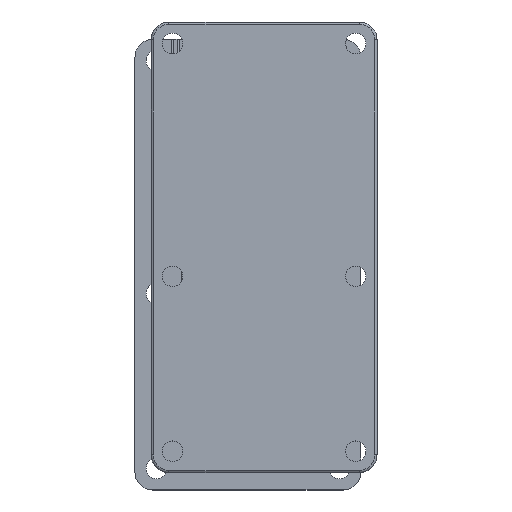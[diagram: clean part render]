
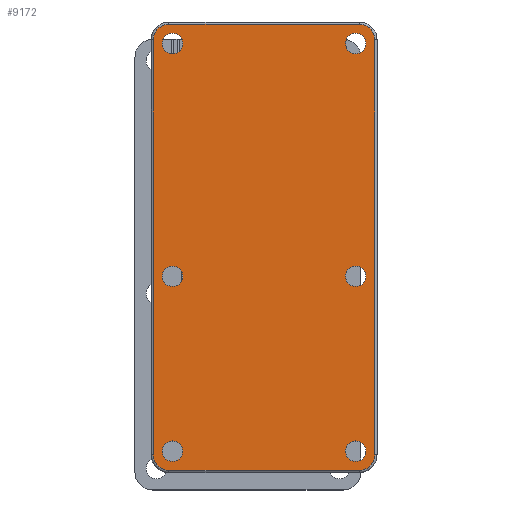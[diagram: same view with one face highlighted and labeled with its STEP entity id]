
A CAD part, top view. The second image highlights one B-rep face of the part: STEP entity #9172.
In plain terms, the highlighted planar face has unit normal (0, 0, 1).
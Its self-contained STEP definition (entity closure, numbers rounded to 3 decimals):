
#223=FACE_BOUND('',#3363,.T.);
#224=FACE_BOUND('',#3364,.T.);
#225=FACE_BOUND('',#3365,.T.);
#226=FACE_BOUND('',#3366,.T.);
#227=FACE_BOUND('',#3367,.T.);
#228=FACE_BOUND('',#3368,.T.);
#682=PLANE('',#9722);
#949=LINE('',#11806,#1873);
#951=LINE('',#11818,#1875);
#953=LINE('',#11830,#1877);
#955=LINE('',#11839,#1879);
#1873=VECTOR('',#10098,10.);
#1875=VECTOR('',#10112,10.);
#1877=VECTOR('',#10126,10.);
#1879=VECTOR('',#10138,10.);
#2844=FACE_OUTER_BOUND('',#3362,.T.);
#3362=EDGE_LOOP('',(#6448,#6449,#6450,#6451,#6452,#6453,#6454,#6455));
#3363=EDGE_LOOP('',(#6456));
#3364=EDGE_LOOP('',(#6457));
#3365=EDGE_LOOP('',(#6458));
#3366=EDGE_LOOP('',(#6459));
#3367=EDGE_LOOP('',(#6460));
#3368=EDGE_LOOP('',(#6461));
#3918=CIRCLE('',#9691,3.5);
#3924=CIRCLE('',#9699,3.5);
#3928=CIRCLE('',#9705,3.5);
#3932=CIRCLE('',#9711,3.5);
#3938=CIRCLE('',#9723,2.3);
#3939=CIRCLE('',#9724,2.3);
#3940=CIRCLE('',#9725,2.3);
#3941=CIRCLE('',#9726,2.3);
#3942=CIRCLE('',#9727,2.3);
#3943=CIRCLE('',#9728,2.3);
#3998=VERTEX_POINT('',#11794);
#3999=VERTEX_POINT('',#11796);
#4001=VERTEX_POINT('',#11802);
#4003=VERTEX_POINT('',#11808);
#4005=VERTEX_POINT('',#11814);
#4007=VERTEX_POINT('',#11820);
#4009=VERTEX_POINT('',#11826);
#4011=VERTEX_POINT('',#11832);
#4082=VERTEX_POINT('',#12103);
#4083=VERTEX_POINT('',#12105);
#4084=VERTEX_POINT('',#12107);
#4085=VERTEX_POINT('',#12109);
#4086=VERTEX_POINT('',#12111);
#4087=VERTEX_POINT('',#12113);
#4929=EDGE_CURVE('',#3998,#3999,#3918,.T.);
#4934=EDGE_CURVE('',#3999,#4001,#949,.T.);
#4937=EDGE_CURVE('',#4001,#4003,#3924,.T.);
#4940=EDGE_CURVE('',#4003,#4005,#951,.T.);
#4943=EDGE_CURVE('',#4005,#4007,#3928,.T.);
#4946=EDGE_CURVE('',#4007,#4009,#953,.T.);
#4949=EDGE_CURVE('',#4009,#4011,#3932,.T.);
#4951=EDGE_CURVE('',#4011,#3998,#955,.T.);
#5025=EDGE_CURVE('',#4082,#4082,#3938,.T.);
#5026=EDGE_CURVE('',#4083,#4083,#3939,.T.);
#5027=EDGE_CURVE('',#4084,#4084,#3940,.T.);
#5028=EDGE_CURVE('',#4085,#4085,#3941,.T.);
#5029=EDGE_CURVE('',#4086,#4086,#3942,.T.);
#5030=EDGE_CURVE('',#4087,#4087,#3943,.T.);
#6448=ORIENTED_EDGE('',*,*,#4929,.F.);
#6449=ORIENTED_EDGE('',*,*,#4951,.F.);
#6450=ORIENTED_EDGE('',*,*,#4949,.F.);
#6451=ORIENTED_EDGE('',*,*,#4946,.F.);
#6452=ORIENTED_EDGE('',*,*,#4943,.F.);
#6453=ORIENTED_EDGE('',*,*,#4940,.F.);
#6454=ORIENTED_EDGE('',*,*,#4937,.F.);
#6455=ORIENTED_EDGE('',*,*,#4934,.F.);
#6456=ORIENTED_EDGE('',*,*,#5025,.T.);
#6457=ORIENTED_EDGE('',*,*,#5026,.T.);
#6458=ORIENTED_EDGE('',*,*,#5027,.T.);
#6459=ORIENTED_EDGE('',*,*,#5028,.T.);
#6460=ORIENTED_EDGE('',*,*,#5029,.T.);
#6461=ORIENTED_EDGE('',*,*,#5030,.T.);
#9172=ADVANCED_FACE('',(#2844,#223,#224,#225,#226,#227,#228),#682,.T.);
#9691=AXIS2_PLACEMENT_3D('',#11797,#10087,#10088);
#9699=AXIS2_PLACEMENT_3D('',#11812,#10105,#10106);
#9705=AXIS2_PLACEMENT_3D('',#11824,#10119,#10120);
#9711=AXIS2_PLACEMENT_3D('',#11836,#10133,#10134);
#9722=AXIS2_PLACEMENT_3D('',#12102,#10196,#10197);
#9723=AXIS2_PLACEMENT_3D('',#12104,#10198,#10199);
#9724=AXIS2_PLACEMENT_3D('',#12106,#10200,#10201);
#9725=AXIS2_PLACEMENT_3D('',#12108,#10202,#10203);
#9726=AXIS2_PLACEMENT_3D('',#12110,#10204,#10205);
#9727=AXIS2_PLACEMENT_3D('',#12112,#10206,#10207);
#9728=AXIS2_PLACEMENT_3D('',#12114,#10208,#10209);
#10087=DIRECTION('center_axis',(0.,0.,-1.));
#10088=DIRECTION('ref_axis',(0.707,0.707,0.));
#10098=DIRECTION('',(0.,-1.,0.));
#10105=DIRECTION('center_axis',(0.,0.,-1.));
#10106=DIRECTION('ref_axis',(0.707,-0.707,0.));
#10112=DIRECTION('',(-1.,0.,0.));
#10119=DIRECTION('center_axis',(0.,0.,-1.));
#10120=DIRECTION('ref_axis',(-0.707,-0.707,0.));
#10126=DIRECTION('',(0.,1.,0.));
#10133=DIRECTION('center_axis',(0.,0.,-1.));
#10134=DIRECTION('ref_axis',(-0.707,0.707,0.));
#10138=DIRECTION('',(1.,0.,0.));
#10196=DIRECTION('center_axis',(0.,0.,1.));
#10197=DIRECTION('ref_axis',(1.,0.,0.));
#10198=DIRECTION('center_axis',(0.,0.,-1.));
#10199=DIRECTION('ref_axis',(1.,0.,0.));
#10200=DIRECTION('center_axis',(0.,0.,-1.));
#10201=DIRECTION('ref_axis',(1.,0.,0.));
#10202=DIRECTION('center_axis',(0.,0.,-1.));
#10203=DIRECTION('ref_axis',(1.,0.,0.));
#10204=DIRECTION('center_axis',(0.,0.,-1.));
#10205=DIRECTION('ref_axis',(1.,0.,0.));
#10206=DIRECTION('center_axis',(0.,0.,-1.));
#10207=DIRECTION('ref_axis',(1.,0.,0.));
#10208=DIRECTION('center_axis',(0.,0.,-1.));
#10209=DIRECTION('ref_axis',(1.,0.,0.));
#11794=CARTESIAN_POINT('',(35.049,109.992,33.292));
#11796=CARTESIAN_POINT('',(38.549,106.492,33.292));
#11797=CARTESIAN_POINT('Origin',(35.049,106.492,33.292));
#11802=CARTESIAN_POINT('',(38.549,13.492,33.292));
#11806=CARTESIAN_POINT('',(38.549,3.492,33.292));
#11808=CARTESIAN_POINT('',(35.049,9.992,33.292));
#11812=CARTESIAN_POINT('Origin',(35.049,13.492,33.292));
#11814=CARTESIAN_POINT('',(-7.605,9.992,33.292));
#11818=CARTESIAN_POINT('',(1.058,9.992,33.292));
#11820=CARTESIAN_POINT('',(-11.105,13.492,33.292));
#11824=CARTESIAN_POINT('Origin',(-7.605,13.492,33.292));
#11826=CARTESIAN_POINT('',(-11.105,106.492,33.292));
#11830=CARTESIAN_POINT('',(-11.105,3.492,33.292));
#11832=CARTESIAN_POINT('',(-7.605,109.992,33.292));
#11836=CARTESIAN_POINT('Origin',(-7.605,106.492,33.292));
#11839=CARTESIAN_POINT('',(1.058,109.992,33.292));
#12102=CARTESIAN_POINT('Origin',(-11.605,3.492,33.292));
#12103=CARTESIAN_POINT('',(-9.105,105.692,33.292));
#12104=CARTESIAN_POINT('Origin',(-6.805,105.692,33.292));
#12105=CARTESIAN_POINT('',(31.949,105.692,33.292));
#12106=CARTESIAN_POINT('Origin',(34.249,105.692,33.292));
#12107=CARTESIAN_POINT('',(-9.105,53.492,33.292));
#12108=CARTESIAN_POINT('Origin',(-6.805,53.492,33.292));
#12109=CARTESIAN_POINT('',(31.949,53.492,33.292));
#12110=CARTESIAN_POINT('Origin',(34.249,53.492,33.292));
#12111=CARTESIAN_POINT('',(31.949,14.292,33.292));
#12112=CARTESIAN_POINT('Origin',(34.249,14.292,33.292));
#12113=CARTESIAN_POINT('',(-9.105,14.292,33.292));
#12114=CARTESIAN_POINT('Origin',(-6.805,14.292,33.292));
